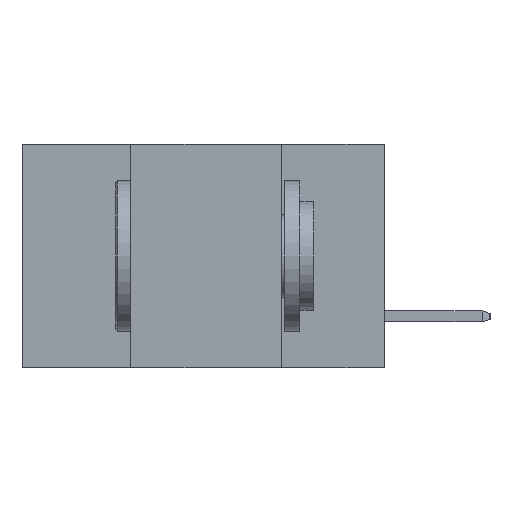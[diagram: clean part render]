
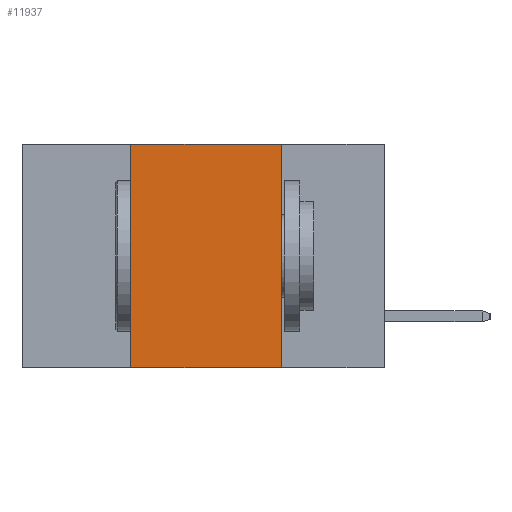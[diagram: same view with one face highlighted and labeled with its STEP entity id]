
A CAD part, left-side view. The second image highlights one B-rep face of the part: STEP entity #11937.
In plain terms, the highlighted planar face has unit normal (-1, 0, 0).
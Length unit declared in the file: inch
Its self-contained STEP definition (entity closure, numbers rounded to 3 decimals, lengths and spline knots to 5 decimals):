
#1680 = CARTESIAN_POINT ( 'NONE',  ( 0., 0.42, 0. ) ) ;
#2388 = LINE ( 'NONE', #21803, #12982 ) ;
#3729 = VECTOR ( 'NONE', #22153, 39.37008 ) ;
#4654 = DIRECTION ( 'NONE',  ( 1., 0., 0. ) ) ;
#4955 = AXIS2_PLACEMENT_3D ( 'NONE', #17153, #4654, #19155 ) ;
#5494 = CARTESIAN_POINT ( 'NONE',  ( 0., 0.17, -0.37 ) ) ;
#8023 = CARTESIAN_POINT ( 'NONE',  ( 0., 0.6, -0.37 ) ) ;
#8194 = VERTEX_POINT ( 'NONE', #5494 ) ;
#8249 = CARTESIAN_POINT ( 'NONE',  ( 0., 0.42, -0.37 ) ) ;
#8917 = EDGE_CURVE ( 'NONE', #18968, #8194, #24812, .T. ) ;
#10035 = VERTEX_POINT ( 'NONE', #11236 ) ;
#11183 = CARTESIAN_POINT ( 'NONE',  ( 0., 0.42, 0. ) ) ;
#11222 = LINE ( 'NONE', #23417, #17319 ) ;
#11236 = CARTESIAN_POINT ( 'NONE',  ( 0., 0.17, 0. ) ) ;
#11688 = EDGE_CURVE ( 'NONE', #18968, #18656, #16059, .T. ) ;
#11937 = ADVANCED_FACE ( 'NONE', ( #26217 ), #24950, .F. ) ;
#12982 = VECTOR ( 'NONE', #19886, 39.37008 ) ;
#13293 = ORIENTED_EDGE ( 'NONE', *, *, #21932, .F. ) ;
#14590 = ORIENTED_EDGE ( 'NONE', *, *, #11688, .F. ) ;
#14881 = EDGE_CURVE ( 'NONE', #18656, #10035, #11222, .T. ) ;
#16059 = LINE ( 'NONE', #1680, #25921 ) ;
#17153 = CARTESIAN_POINT ( 'NONE',  ( 0., 0.6, 0. ) ) ;
#17319 = VECTOR ( 'NONE', #19514, 39.37008 ) ;
#18397 = DIRECTION ( 'NONE',  ( 0., 0., 1. ) ) ;
#18656 = VERTEX_POINT ( 'NONE', #11183 ) ;
#18689 = ORIENTED_EDGE ( 'NONE', *, *, #14881, .F. ) ;
#18968 = VERTEX_POINT ( 'NONE', #8249 ) ;
#19155 = DIRECTION ( 'NONE',  ( 0., 0., -1. ) ) ;
#19514 = DIRECTION ( 'NONE',  ( 0., -1., 0. ) ) ;
#19886 = DIRECTION ( 'NONE',  ( 0., 0., -1. ) ) ;
#19902 = ORIENTED_EDGE ( 'NONE', *, *, #8917, .T. ) ;
#21803 = CARTESIAN_POINT ( 'NONE',  ( 0., 0.17, 0. ) ) ;
#21932 = EDGE_CURVE ( 'NONE', #10035, #8194, #2388, .T. ) ;
#22153 = DIRECTION ( 'NONE',  ( 0., -1., 0. ) ) ;
#23417 = CARTESIAN_POINT ( 'NONE',  ( 0., 0.6, 0. ) ) ;
#24812 = LINE ( 'NONE', #8023, #3729 ) ;
#24950 = PLANE ( 'NONE',  #4955 ) ;
#25921 = VECTOR ( 'NONE', #18397, 39.37008 ) ;
#26217 = FACE_OUTER_BOUND ( 'NONE', #26297, .T. ) ;
#26297 = EDGE_LOOP ( 'NONE', ( #13293, #18689, #14590, #19902 ) ) ;
